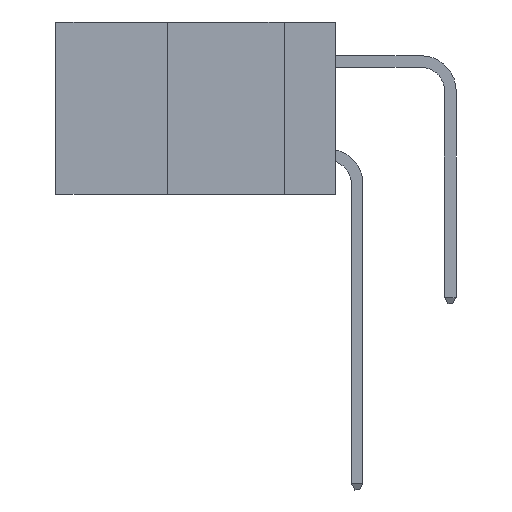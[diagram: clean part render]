
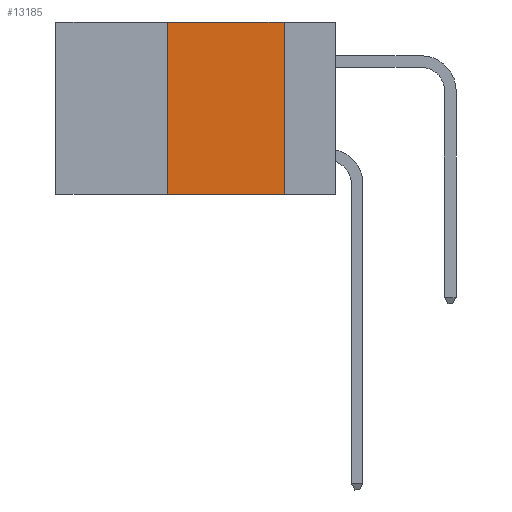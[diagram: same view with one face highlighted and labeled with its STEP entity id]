
A CAD part, left-side view. The second image highlights one B-rep face of the part: STEP entity #13185.
In plain terms, the highlighted planar face has unit normal (-1, 0, 0).
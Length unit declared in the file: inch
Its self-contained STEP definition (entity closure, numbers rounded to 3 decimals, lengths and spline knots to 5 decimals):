
#70 = LINE ( 'NONE', #11743, #11700 ) ;
#621 = DIRECTION ( 'NONE',  ( 0., -1., 0. ) ) ;
#1192 = VECTOR ( 'NONE', #12136, 39.37008 ) ;
#1335 = EDGE_CURVE ( 'NONE', #6956, #13882, #9497, .T. ) ;
#1341 = VERTEX_POINT ( 'NONE', #12938 ) ;
#1709 = CARTESIAN_POINT ( 'NONE',  ( 0., 0.6, 0. ) ) ;
#1896 = CARTESIAN_POINT ( 'NONE',  ( 0., 0.11, -0.37 ) ) ;
#2071 = DIRECTION ( 'NONE',  ( 0., 0., -1. ) ) ;
#2789 = DIRECTION ( 'NONE',  ( 1., 0., 0. ) ) ;
#2848 = CARTESIAN_POINT ( 'NONE',  ( 0., 0.6, 0. ) ) ;
#2884 = CARTESIAN_POINT ( 'NONE',  ( 0., 0.36, 0. ) ) ;
#3193 = VECTOR ( 'NONE', #6048, 39.37008 ) ;
#4441 = ORIENTED_EDGE ( 'NONE', *, *, #13395, .F. ) ;
#4624 = CARTESIAN_POINT ( 'NONE',  ( 0., 0.36, -0.37 ) ) ;
#5636 = FACE_OUTER_BOUND ( 'NONE', #12948, .T. ) ;
#6048 = DIRECTION ( 'NONE',  ( 0., -1., 0. ) ) ;
#6093 = PLANE ( 'NONE',  #9153 ) ;
#6956 = VERTEX_POINT ( 'NONE', #4624 ) ;
#7079 = CARTESIAN_POINT ( 'NONE',  ( 0., 0.6, -0.37 ) ) ;
#8185 = DIRECTION ( 'NONE',  ( 0., 0., -1. ) ) ;
#8339 = ORIENTED_EDGE ( 'NONE', *, *, #9981, .F. ) ;
#8924 = ORIENTED_EDGE ( 'NONE', *, *, #11219, .F. ) ;
#9024 = LINE ( 'NONE', #2848, #3193 ) ;
#9153 = AXIS2_PLACEMENT_3D ( 'NONE', #1709, #2789, #8185 ) ;
#9397 = LINE ( 'NONE', #2884, #1192 ) ;
#9497 = LINE ( 'NONE', #7079, #12582 ) ;
#9981 = EDGE_CURVE ( 'NONE', #6956, #13547, #9397, .T. ) ;
#10744 = ORIENTED_EDGE ( 'NONE', *, *, #1335, .T. ) ;
#11038 = CARTESIAN_POINT ( 'NONE',  ( 0., 0.36, 0. ) ) ;
#11219 = EDGE_CURVE ( 'NONE', #13547, #1341, #9024, .T. ) ;
#11700 = VECTOR ( 'NONE', #2071, 39.37008 ) ;
#11743 = CARTESIAN_POINT ( 'NONE',  ( 0., 0.11, 0. ) ) ;
#12136 = DIRECTION ( 'NONE',  ( 0., 0., 1. ) ) ;
#12582 = VECTOR ( 'NONE', #621, 39.37008 ) ;
#12938 = CARTESIAN_POINT ( 'NONE',  ( 0., 0.11, 0. ) ) ;
#12948 = EDGE_LOOP ( 'NONE', ( #4441, #8924, #8339, #10744 ) ) ;
#13185 = ADVANCED_FACE ( 'NONE', ( #5636 ), #6093, .F. ) ;
#13395 = EDGE_CURVE ( 'NONE', #1341, #13882, #70, .T. ) ;
#13547 = VERTEX_POINT ( 'NONE', #11038 ) ;
#13882 = VERTEX_POINT ( 'NONE', #1896 ) ;
